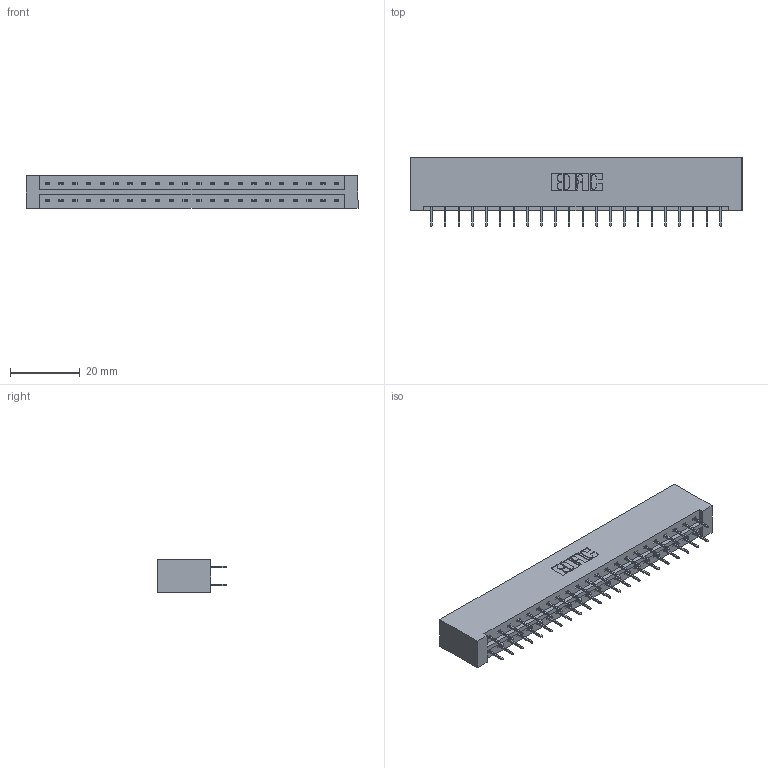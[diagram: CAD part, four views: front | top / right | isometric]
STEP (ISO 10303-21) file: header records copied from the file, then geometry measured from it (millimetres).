
FILE_DESCRIPTION (( 'STEP AP203' ), '1' );
FILE_NAME ('833-044-524-201.STEP', '2020-06-04T01:04:18', ( '' ), ( '' ), 'SwSTEP 2.0', 'SolidWorks 2020', '' );
FILE_SCHEMA (( 'CONFIG_CONTROL_DESIGN' ));
Length unit declared in the file: inch
Products named in the file (3): 345-292-001_345-293-124; 833 Part_Lugless; 833-044-524-201
Assembly tree (45 placements, depth 2):
  833-044-524-201
    833 Part_Lugless
    345-292-001_345-293-124  x44
Bounding box: 95.43 x 19.69 x 9.4 mm (x, y, z)
Volume: 10121.2 mm3; surface area: 11575.4 mm2
Topology: 45 solids, 45 shells, 2570 faces, 7283 edges, 4678 vertices
Faces by surface type: plane 1914, cylinder 656
Entity records: 16537 total; most frequent: CARTESIAN_POINT 2762, ORIENTED_EDGE 2698, DIRECTION 2389, EDGE_CURVE 1349, LINE 1233, VECTOR 1233, VERTEX_POINT 894, AXIS2_PLACEMENT_3D 578
